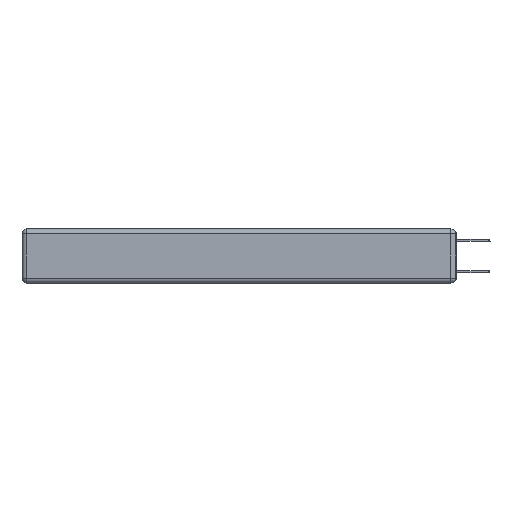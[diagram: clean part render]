
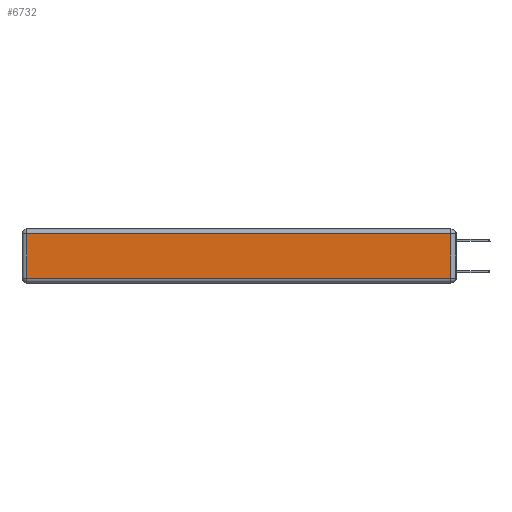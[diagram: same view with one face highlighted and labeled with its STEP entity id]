
A CAD part, left-side view. The second image highlights one B-rep face of the part: STEP entity #6732.
In plain terms, the highlighted planar face has unit normal (-1, 0, 0).
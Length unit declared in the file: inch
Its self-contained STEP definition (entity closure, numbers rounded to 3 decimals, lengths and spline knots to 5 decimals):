
#86 = LINE ( 'NONE', #313, #10138 ) ;
#136 = CARTESIAN_POINT ( 'NONE',  ( 0., 0.03, -0.313 ) ) ;
#313 = CARTESIAN_POINT ( 'NONE',  ( 0., 0., -0.313 ) ) ;
#1496 = DIRECTION ( 'NONE',  ( -1., 0., 0. ) ) ;
#2183 = VERTEX_POINT ( 'NONE', #2579 ) ;
#2283 = VERTEX_POINT ( 'NONE', #136 ) ;
#2579 = CARTESIAN_POINT ( 'NONE',  ( 0., 2.72, -0.03 ) ) ;
#3464 = VECTOR ( 'NONE', #14748, 39.37008 ) ;
#3511 = LINE ( 'NONE', #12955, #14992 ) ;
#3570 = VECTOR ( 'NONE', #13752, 39.37008 ) ;
#3610 = EDGE_LOOP ( 'NONE', ( #5125, #6325, #10529, #5000 ) ) ;
#4369 = LINE ( 'NONE', #9091, #3570 ) ;
#4970 = EDGE_CURVE ( 'NONE', #9613, #2183, #11409, .T. ) ;
#5000 = ORIENTED_EDGE ( 'NONE', *, *, #8924, .T. ) ;
#5125 = ORIENTED_EDGE ( 'NONE', *, *, #10829, .T. ) ;
#6325 = ORIENTED_EDGE ( 'NONE', *, *, #14620, .T. ) ;
#6378 = FACE_OUTER_BOUND ( 'NONE', #3610, .T. ) ;
#6699 = CARTESIAN_POINT ( 'NONE',  ( 0., 2.72, -0.313 ) ) ;
#6732 = ADVANCED_FACE ( 'NONE', ( #6378 ), #13487, .T. ) ;
#7008 = AXIS2_PLACEMENT_3D ( 'NONE', #12292, #1496, #7631 ) ;
#7105 = DIRECTION ( 'NONE',  ( 0., 0., 1. ) ) ;
#7312 = DIRECTION ( 'NONE',  ( 0., -1., 0. ) ) ;
#7631 = DIRECTION ( 'NONE',  ( 0., 0., 1. ) ) ;
#7756 = CARTESIAN_POINT ( 'NONE',  ( 0., 0.03, -0.03 ) ) ;
#8139 = VERTEX_POINT ( 'NONE', #6699 ) ;
#8924 = EDGE_CURVE ( 'NONE', #2183, #8139, #4369, .T. ) ;
#9091 = CARTESIAN_POINT ( 'NONE',  ( 0., 2.72, -0.343 ) ) ;
#9613 = VERTEX_POINT ( 'NONE', #7756 ) ;
#10138 = VECTOR ( 'NONE', #7312, 39.37008 ) ;
#10152 = CARTESIAN_POINT ( 'NONE',  ( 0., 2.75, -0.03 ) ) ;
#10529 = ORIENTED_EDGE ( 'NONE', *, *, #4970, .T. ) ;
#10829 = EDGE_CURVE ( 'NONE', #8139, #2283, #86, .T. ) ;
#11409 = LINE ( 'NONE', #10152, #3464 ) ;
#12292 = CARTESIAN_POINT ( 'NONE',  ( 0., 0., -0.343 ) ) ;
#12955 = CARTESIAN_POINT ( 'NONE',  ( 0., 0.03, -0.343 ) ) ;
#13487 = PLANE ( 'NONE',  #7008 ) ;
#13752 = DIRECTION ( 'NONE',  ( 0., 0., -1. ) ) ;
#14620 = EDGE_CURVE ( 'NONE', #2283, #9613, #3511, .T. ) ;
#14748 = DIRECTION ( 'NONE',  ( 0., 1., 0. ) ) ;
#14992 = VECTOR ( 'NONE', #7105, 39.37008 ) ;
